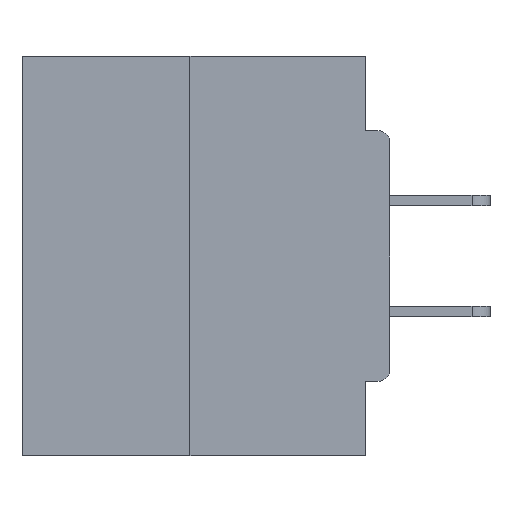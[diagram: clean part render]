
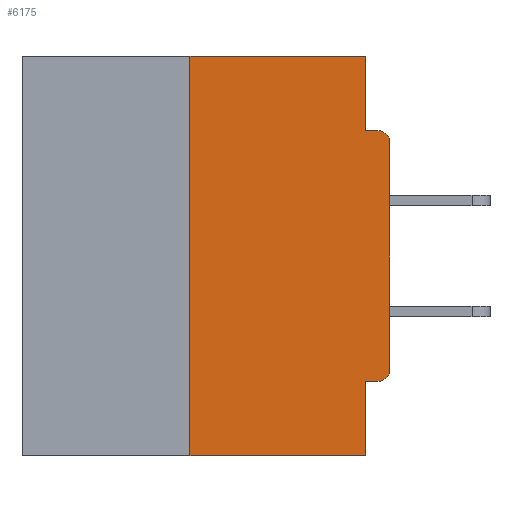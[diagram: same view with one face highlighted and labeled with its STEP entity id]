
A CAD part, left-side view. The second image highlights one B-rep face of the part: STEP entity #6175.
In plain terms, the highlighted planar face has unit normal (-1, 0, 0).
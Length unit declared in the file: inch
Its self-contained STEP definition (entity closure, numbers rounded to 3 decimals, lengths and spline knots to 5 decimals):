
#142 = VERTEX_POINT ( 'NONE', #38547 ) ;
#304 = CIRCLE ( 'NONE', #28050, 0.015 ) ;
#616 = DIRECTION ( 'NONE',  ( 0., 0., -1. ) ) ;
#1393 = EDGE_CURVE ( 'NONE', #30312, #3960, #21138, .T. ) ;
#1800 = EDGE_CURVE ( 'NONE', #25986, #33120, #9398, .T. ) ;
#1805 = CARTESIAN_POINT ( 'NONE',  ( 0., 0.031, -0.5 ) ) ;
#2829 = EDGE_CURVE ( 'NONE', #4477, #18828, #24708, .T. ) ;
#2961 = CARTESIAN_POINT ( 'NONE',  ( 0., 0.015, -0.0935 ) ) ;
#3960 = VERTEX_POINT ( 'NONE', #1805 ) ;
#4477 = VERTEX_POINT ( 'NONE', #31106 ) ;
#4573 = EDGE_CURVE ( 'NONE', #11503, #18828, #304, .T. ) ;
#5603 = VECTOR ( 'NONE', #18443, 39.37008 ) ;
#6175 = ADVANCED_FACE ( 'NONE', ( #22020 ), #27858, .F. ) ;
#6764 = VECTOR ( 'NONE', #37281, 39.37008 ) ;
#6981 = ORIENTED_EDGE ( 'NONE', *, *, #23821, .F. ) ;
#7100 = ORIENTED_EDGE ( 'NONE', *, *, #12148, .F. ) ;
#7143 = CARTESIAN_POINT ( 'NONE',  ( 0., 0.46, 0. ) ) ;
#7600 = CARTESIAN_POINT ( 'NONE',  ( 0., 0.015, -0.1085 ) ) ;
#7755 = LINE ( 'NONE', #7143, #38562 ) ;
#8233 = ORIENTED_EDGE ( 'NONE', *, *, #4573, .T. ) ;
#9398 = LINE ( 'NONE', #35325, #15953 ) ;
#9434 = VECTOR ( 'NONE', #15724, 39.37008 ) ;
#9671 = CARTESIAN_POINT ( 'NONE',  ( 0., 0., -0.0935 ) ) ;
#9996 = CARTESIAN_POINT ( 'NONE',  ( 0., 0.46, 0. ) ) ;
#10055 = CARTESIAN_POINT ( 'NONE',  ( 0., 0., -0.1085 ) ) ;
#10111 = AXIS2_PLACEMENT_3D ( 'NONE', #9996, #33893, #36361 ) ;
#11503 = VERTEX_POINT ( 'NONE', #10055 ) ;
#12042 = DIRECTION ( 'NONE',  ( 0., 0., 1. ) ) ;
#12148 = EDGE_CURVE ( 'NONE', #33120, #3960, #21704, .T. ) ;
#13219 = EDGE_CURVE ( 'NONE', #30312, #35096, #31064, .T. ) ;
#13870 = DIRECTION ( 'NONE',  ( -1., 0., 0. ) ) ;
#14043 = CARTESIAN_POINT ( 'NONE',  ( 0., 0.25, 0. ) ) ;
#14192 = EDGE_CURVE ( 'NONE', #142, #11503, #20724, .T. ) ;
#14700 = ORIENTED_EDGE ( 'NONE', *, *, #22267, .T. ) ;
#15465 = CARTESIAN_POINT ( 'NONE',  ( 0., 0.25, 0. ) ) ;
#15724 = DIRECTION ( 'NONE',  ( 0., -1., 0. ) ) ;
#15953 = VECTOR ( 'NONE', #35583, 39.37008 ) ;
#16119 = CARTESIAN_POINT ( 'NONE',  ( 0., 0.46, -0.5 ) ) ;
#16915 = EDGE_LOOP ( 'NONE', ( #37816, #31558, #17769, #7100, #19909, #14700, #26640, #8233, #22220, #6981 ) ) ;
#17769 = ORIENTED_EDGE ( 'NONE', *, *, #1393, .T. ) ;
#18217 = DIRECTION ( 'NONE',  ( -1., 0., 0. ) ) ;
#18443 = DIRECTION ( 'NONE',  ( 0., -1., 0. ) ) ;
#18608 = VECTOR ( 'NONE', #24937, 39.37008 ) ;
#18667 = CIRCLE ( 'NONE', #34229, 0.015 ) ;
#18828 = VERTEX_POINT ( 'NONE', #2961 ) ;
#19340 = DIRECTION ( 'NONE',  ( 0., 0., -1. ) ) ;
#19414 = DIRECTION ( 'NONE',  ( 0., -1., 0. ) ) ;
#19909 = ORIENTED_EDGE ( 'NONE', *, *, #1800, .F. ) ;
#20724 = LINE ( 'NONE', #32575, #23487 ) ;
#21138 = LINE ( 'NONE', #16119, #9434 ) ;
#21670 = VECTOR ( 'NONE', #34526, 39.37008 ) ;
#21704 = LINE ( 'NONE', #28563, #6764 ) ;
#21867 = CARTESIAN_POINT ( 'NONE',  ( 0., 0.015, -0.4065 ) ) ;
#22020 = FACE_OUTER_BOUND ( 'NONE', #16915, .T. ) ;
#22220 = ORIENTED_EDGE ( 'NONE', *, *, #2829, .F. ) ;
#22267 = EDGE_CURVE ( 'NONE', #25986, #142, #18667, .T. ) ;
#22328 = LINE ( 'NONE', #36824, #18608 ) ;
#22650 = CARTESIAN_POINT ( 'NONE',  ( 0., 0.031, 0. ) ) ;
#23487 = VECTOR ( 'NONE', #12042, 39.37008 ) ;
#23821 = EDGE_CURVE ( 'NONE', #34913, #4477, #22328, .T. ) ;
#24708 = LINE ( 'NONE', #9671, #5603 ) ;
#24937 = DIRECTION ( 'NONE',  ( 0., 0., -1. ) ) ;
#25986 = VERTEX_POINT ( 'NONE', #21867 ) ;
#26640 = ORIENTED_EDGE ( 'NONE', *, *, #14192, .T. ) ;
#27858 = PLANE ( 'NONE',  #10111 ) ;
#28050 = AXIS2_PLACEMENT_3D ( 'NONE', #7600, #13870, #19340 ) ;
#28563 = CARTESIAN_POINT ( 'NONE',  ( 0., 0.031, -0.5 ) ) ;
#30312 = VERTEX_POINT ( 'NONE', #34643 ) ;
#31064 = LINE ( 'NONE', #14043, #21670 ) ;
#31106 = CARTESIAN_POINT ( 'NONE',  ( 0., 0.031, -0.0935 ) ) ;
#31505 = EDGE_CURVE ( 'NONE', #35096, #34913, #7755, .T. ) ;
#31558 = ORIENTED_EDGE ( 'NONE', *, *, #13219, .F. ) ;
#32575 = CARTESIAN_POINT ( 'NONE',  ( 0., 0., 0. ) ) ;
#32694 = CARTESIAN_POINT ( 'NONE',  ( 0., 0.031, -0.4065 ) ) ;
#33120 = VERTEX_POINT ( 'NONE', #32694 ) ;
#33893 = DIRECTION ( 'NONE',  ( 1., 0., 0. ) ) ;
#34229 = AXIS2_PLACEMENT_3D ( 'NONE', #36100, #18217, #616 ) ;
#34526 = DIRECTION ( 'NONE',  ( 0., 0., 1. ) ) ;
#34643 = CARTESIAN_POINT ( 'NONE',  ( 0., 0.25, -0.5 ) ) ;
#34913 = VERTEX_POINT ( 'NONE', #22650 ) ;
#35096 = VERTEX_POINT ( 'NONE', #15465 ) ;
#35325 = CARTESIAN_POINT ( 'NONE',  ( 0., 0., -0.4065 ) ) ;
#35583 = DIRECTION ( 'NONE',  ( 0., 1., 0. ) ) ;
#36100 = CARTESIAN_POINT ( 'NONE',  ( 0., 0.015, -0.3915 ) ) ;
#36361 = DIRECTION ( 'NONE',  ( 0., 0., -1. ) ) ;
#36824 = CARTESIAN_POINT ( 'NONE',  ( 0., 0.031, 0. ) ) ;
#37281 = DIRECTION ( 'NONE',  ( 0., 0., -1. ) ) ;
#37816 = ORIENTED_EDGE ( 'NONE', *, *, #31505, .F. ) ;
#38547 = CARTESIAN_POINT ( 'NONE',  ( 0., 0., -0.3915 ) ) ;
#38562 = VECTOR ( 'NONE', #19414, 39.37008 ) ;
